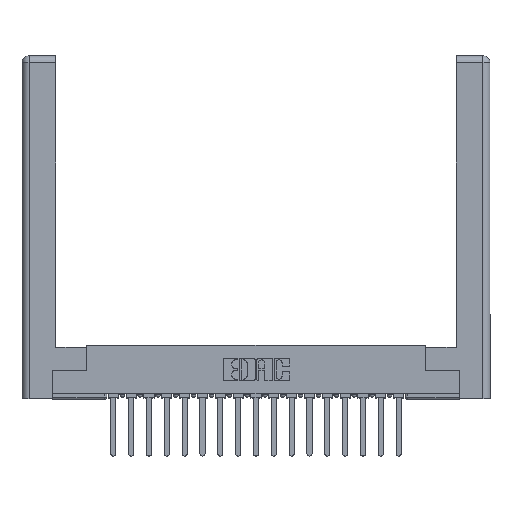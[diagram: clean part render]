
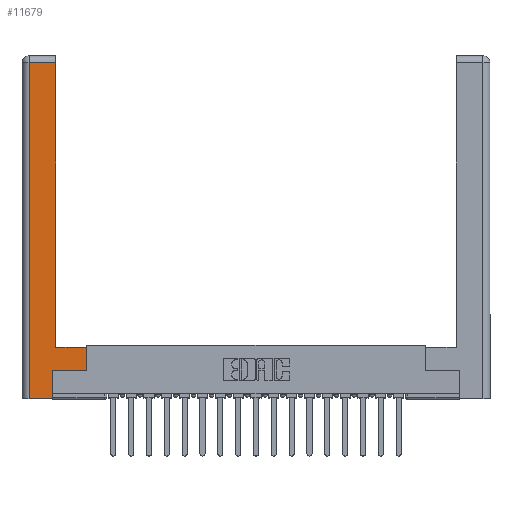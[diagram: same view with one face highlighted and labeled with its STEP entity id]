
A CAD part, top view. The second image highlights one B-rep face of the part: STEP entity #11679.
In plain terms, the highlighted planar face has unit normal (0, 0, 1).
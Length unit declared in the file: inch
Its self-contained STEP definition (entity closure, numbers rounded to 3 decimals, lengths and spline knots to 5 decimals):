
#285 = LINE ( 'NONE', #1289, #15263 ) ;
#767 = LINE ( 'NONE', #4009, #4291 ) ;
#784 = VERTEX_POINT ( 'NONE', #7255 ) ;
#947 = CARTESIAN_POINT ( 'NONE',  ( 0.0615, 0., 0. ) ) ;
#1289 = CARTESIAN_POINT ( 'NONE',  ( 0.295, 0.45, 0. ) ) ;
#1507 = DIRECTION ( 'NONE',  ( 0., 0., -1. ) ) ;
#2568 = ORIENTED_EDGE ( 'NONE', *, *, #3111, .T. ) ;
#3111 = EDGE_CURVE ( 'NONE', #11955, #7259, #18286, .T. ) ;
#3260 = EDGE_CURVE ( 'NONE', #6734, #12768, #17768, .T. ) ;
#3614 = AXIS2_PLACEMENT_3D ( 'NONE', #7921, #1507, #4945 ) ;
#3795 = CARTESIAN_POINT ( 'NONE',  ( 0.295, 2.94, 0. ) ) ;
#4009 = CARTESIAN_POINT ( 'NONE',  ( 0.565, 0.45, 0. ) ) ;
#4291 = VECTOR ( 'NONE', #14131, 39.37008 ) ;
#4945 = DIRECTION ( 'NONE',  ( -1., 0., 0. ) ) ;
#5688 = VECTOR ( 'NONE', #6456, 39.37008 ) ;
#6037 = VECTOR ( 'NONE', #7016, 39.37008 ) ;
#6209 = LINE ( 'NONE', #9416, #5688 ) ;
#6456 = DIRECTION ( 'NONE',  ( -1., 0., 0. ) ) ;
#6734 = VERTEX_POINT ( 'NONE', #7592 ) ;
#6784 = ORIENTED_EDGE ( 'NONE', *, *, #17787, .T. ) ;
#7016 = DIRECTION ( 'NONE',  ( 0., -1., 0. ) ) ;
#7255 = CARTESIAN_POINT ( 'NONE',  ( 0.565, 0.45, 0. ) ) ;
#7259 = VERTEX_POINT ( 'NONE', #947 ) ;
#7465 = CARTESIAN_POINT ( 'NONE',  ( 0.265, 0., 0. ) ) ;
#7592 = CARTESIAN_POINT ( 'NONE',  ( 0.295, 0.45, 0. ) ) ;
#7921 = CARTESIAN_POINT ( 'NONE',  ( 0., 0., 0. ) ) ;
#8063 = PLANE ( 'NONE',  #3614 ) ;
#8497 = VERTEX_POINT ( 'NONE', #9476 ) ;
#8716 = CARTESIAN_POINT ( 'NONE',  ( 0.265, 0., 0. ) ) ;
#8748 = EDGE_CURVE ( 'NONE', #12768, #11955, #6209, .T. ) ;
#9370 = FACE_OUTER_BOUND ( 'NONE', #15583, .T. ) ;
#9394 = VERTEX_POINT ( 'NONE', #8716 ) ;
#9416 = CARTESIAN_POINT ( 'NONE',  ( 0.0615, 2.94, 0. ) ) ;
#9476 = CARTESIAN_POINT ( 'NONE',  ( 0.565, 0.245, 0. ) ) ;
#10221 = EDGE_CURVE ( 'NONE', #14771, #8497, #16093, .T. ) ;
#11107 = ORIENTED_EDGE ( 'NONE', *, *, #12383, .T. ) ;
#11314 = EDGE_CURVE ( 'NONE', #9394, #14771, #20865, .T. ) ;
#11526 = LINE ( 'NONE', #7465, #16149 ) ;
#11679 = ADVANCED_FACE ( 'NONE', ( #9370 ), #8063, .F. ) ;
#11783 = ORIENTED_EDGE ( 'NONE', *, *, #11314, .T. ) ;
#11825 = ORIENTED_EDGE ( 'NONE', *, *, #3260, .T. ) ;
#11955 = VERTEX_POINT ( 'NONE', #18409 ) ;
#12222 = CARTESIAN_POINT ( 'NONE',  ( 0.265, 0.245, 0. ) ) ;
#12383 = EDGE_CURVE ( 'NONE', #784, #6734, #285, .T. ) ;
#12439 = EDGE_CURVE ( 'NONE', #8497, #784, #767, .T. ) ;
#12520 = ORIENTED_EDGE ( 'NONE', *, *, #8748, .T. ) ;
#12552 = DIRECTION ( 'NONE',  ( -1., 0., 0. ) ) ;
#12768 = VERTEX_POINT ( 'NONE', #3795 ) ;
#13778 = CARTESIAN_POINT ( 'NONE',  ( 0.295, 3., 0. ) ) ;
#14025 = DIRECTION ( 'NONE',  ( 1., 0., 0. ) ) ;
#14028 = ORIENTED_EDGE ( 'NONE', *, *, #12439, .T. ) ;
#14131 = DIRECTION ( 'NONE',  ( 0., 1., 0. ) ) ;
#14189 = DIRECTION ( 'NONE',  ( 1., 0., 0. ) ) ;
#14771 = VERTEX_POINT ( 'NONE', #15466 ) ;
#15263 = VECTOR ( 'NONE', #12552, 39.37008 ) ;
#15466 = CARTESIAN_POINT ( 'NONE',  ( 0.265, 0.245, 0. ) ) ;
#15495 = DIRECTION ( 'NONE',  ( 0., 1., 0. ) ) ;
#15583 = EDGE_LOOP ( 'NONE', ( #11825, #12520, #2568, #6784, #11783, #20035, #14028, #11107 ) ) ;
#15652 = DIRECTION ( 'NONE',  ( 0., 1., 0. ) ) ;
#16093 = LINE ( 'NONE', #20732, #20150 ) ;
#16149 = VECTOR ( 'NONE', #14025, 39.37008 ) ;
#16573 = VECTOR ( 'NONE', #15652, 39.37008 ) ;
#17768 = LINE ( 'NONE', #13778, #19538 ) ;
#17787 = EDGE_CURVE ( 'NONE', #7259, #9394, #11526, .T. ) ;
#18286 = LINE ( 'NONE', #20033, #6037 ) ;
#18409 = CARTESIAN_POINT ( 'NONE',  ( 0.0615, 2.94, 0. ) ) ;
#19538 = VECTOR ( 'NONE', #15495, 39.37008 ) ;
#20033 = CARTESIAN_POINT ( 'NONE',  ( 0.0615, 0., 0. ) ) ;
#20035 = ORIENTED_EDGE ( 'NONE', *, *, #10221, .T. ) ;
#20150 = VECTOR ( 'NONE', #14189, 39.37008 ) ;
#20732 = CARTESIAN_POINT ( 'NONE',  ( 0.565, 0.245, 0. ) ) ;
#20865 = LINE ( 'NONE', #12222, #16573 ) ;
